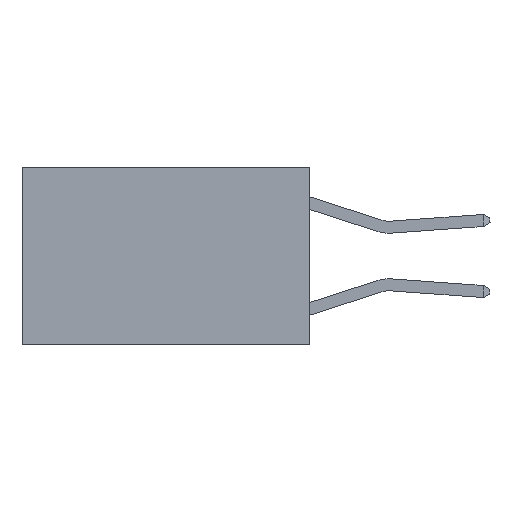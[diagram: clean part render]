
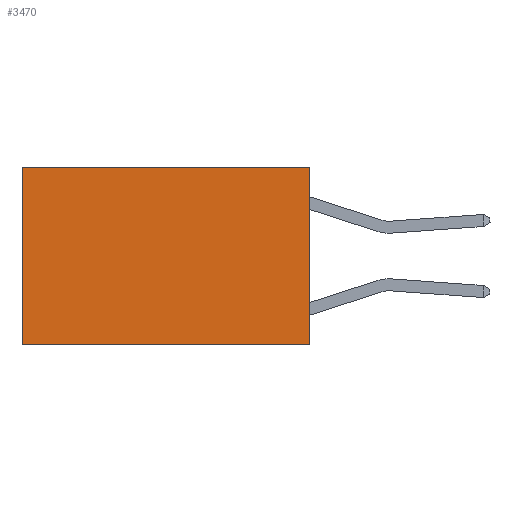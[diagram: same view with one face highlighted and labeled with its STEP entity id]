
A CAD part, left-side view. The second image highlights one B-rep face of the part: STEP entity #3470.
In plain terms, the highlighted planar face has unit normal (-1, 0, 0).
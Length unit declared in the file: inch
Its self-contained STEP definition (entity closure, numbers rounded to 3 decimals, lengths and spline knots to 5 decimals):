
#154 = DIRECTION ( 'NONE',  ( 0., 1., 0. ) ) ;
#665 = DIRECTION ( 'NONE',  ( 0., 0., -1. ) ) ;
#770 = VERTEX_POINT ( 'NONE', #10614 ) ;
#1066 = CARTESIAN_POINT ( 'NONE',  ( 0.2625, 0., 0. ) ) ;
#1722 = VECTOR ( 'NONE', #12211, 39.37008 ) ;
#2676 = VECTOR ( 'NONE', #154, 39.37008 ) ;
#3202 = CARTESIAN_POINT ( 'NONE',  ( 0.2625, 0., -0.37 ) ) ;
#3470 = ADVANCED_FACE ( 'NONE', ( #13485 ), #9838, .F. ) ;
#3479 = CARTESIAN_POINT ( 'NONE',  ( 0.2625, 0., 0. ) ) ;
#4194 = ORIENTED_EDGE ( 'NONE', *, *, #7428, .T. ) ;
#4212 = ORIENTED_EDGE ( 'NONE', *, *, #13878, .F. ) ;
#4243 = DIRECTION ( 'NONE',  ( 0., 0., -1. ) ) ;
#4763 = ORIENTED_EDGE ( 'NONE', *, *, #12167, .F. ) ;
#4830 = ORIENTED_EDGE ( 'NONE', *, *, #6741, .T. ) ;
#4892 = VECTOR ( 'NONE', #665, 39.37008 ) ;
#5041 = CARTESIAN_POINT ( 'NONE',  ( 0.2625, 0., 0. ) ) ;
#6050 = LINE ( 'NONE', #7916, #16645 ) ;
#6741 = EDGE_CURVE ( 'NONE', #10885, #770, #16461, .T. ) ;
#6904 = CARTESIAN_POINT ( 'NONE',  ( 0.2625, 0.6, -0.37 ) ) ;
#7428 = EDGE_CURVE ( 'NONE', #770, #17273, #6050, .T. ) ;
#7916 = CARTESIAN_POINT ( 'NONE',  ( 0.2625, 0.6, 0. ) ) ;
#8359 = DIRECTION ( 'NONE',  ( 1., 0., 0. ) ) ;
#9824 = AXIS2_PLACEMENT_3D ( 'NONE', #12568, #8359, #4243 ) ;
#9838 = PLANE ( 'NONE',  #9824 ) ;
#10075 = LINE ( 'NONE', #12698, #2676 ) ;
#10614 = CARTESIAN_POINT ( 'NONE',  ( 0.2625, 0.6, 0. ) ) ;
#10885 = VERTEX_POINT ( 'NONE', #5041 ) ;
#11361 = VERTEX_POINT ( 'NONE', #3202 ) ;
#12127 = DIRECTION ( 'NONE',  ( 0., 0., -1. ) ) ;
#12167 = EDGE_CURVE ( 'NONE', #10885, #11361, #12305, .T. ) ;
#12211 = DIRECTION ( 'NONE',  ( 0., 1., 0. ) ) ;
#12305 = LINE ( 'NONE', #3479, #4892 ) ;
#12568 = CARTESIAN_POINT ( 'NONE',  ( 0.2625, 0., 0. ) ) ;
#12698 = CARTESIAN_POINT ( 'NONE',  ( 0.2625, 0., -0.37 ) ) ;
#13485 = FACE_OUTER_BOUND ( 'NONE', #15175, .T. ) ;
#13878 = EDGE_CURVE ( 'NONE', #11361, #17273, #10075, .T. ) ;
#15175 = EDGE_LOOP ( 'NONE', ( #4194, #4212, #4763, #4830 ) ) ;
#16461 = LINE ( 'NONE', #1066, #1722 ) ;
#16645 = VECTOR ( 'NONE', #12127, 39.37008 ) ;
#17273 = VERTEX_POINT ( 'NONE', #6904 ) ;
